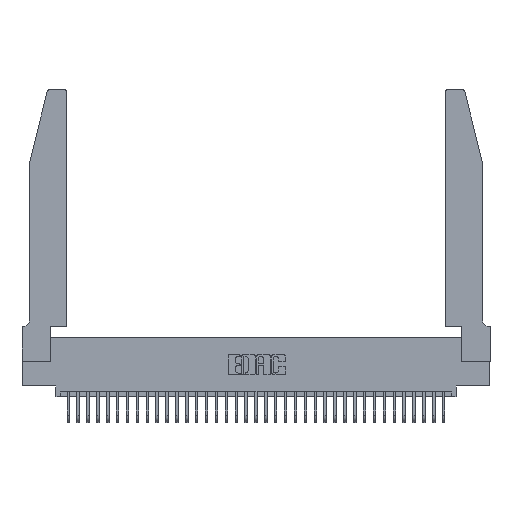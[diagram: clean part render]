
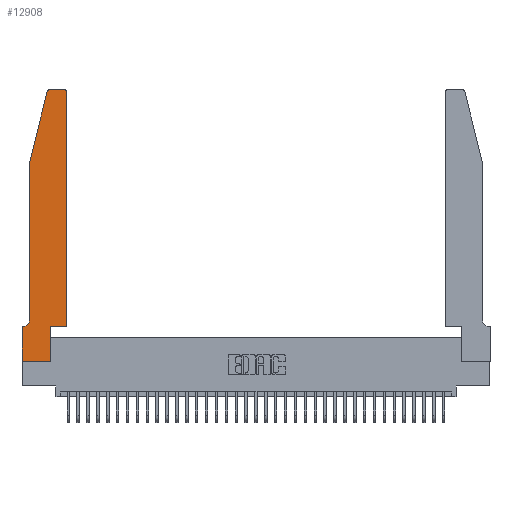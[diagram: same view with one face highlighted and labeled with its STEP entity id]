
A CAD part, top view. The second image highlights one B-rep face of the part: STEP entity #12908.
In plain terms, the highlighted planar face has unit normal (0, 0, 1).
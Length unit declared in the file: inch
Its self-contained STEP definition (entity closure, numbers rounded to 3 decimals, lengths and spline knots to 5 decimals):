
#141 = VERTEX_POINT ( 'NONE', #36667 ) ;
#667 = VERTEX_POINT ( 'NONE', #1172 ) ;
#768 = DIRECTION ( 'NONE',  ( -0.239, -0.971, 0. ) ) ;
#1172 = CARTESIAN_POINT ( 'NONE',  ( 0.4505, 2.72, 0.37 ) ) ;
#1260 = VECTOR ( 'NONE', #20683, 39.37008 ) ;
#2065 = CARTESIAN_POINT ( 'NONE',  ( 0.4205, 2.75, 0.37 ) ) ;
#2400 = EDGE_CURVE ( 'NONE', #3480, #141, #33584, .T. ) ;
#2544 = DIRECTION ( 'NONE',  ( 1., 0., 0. ) ) ;
#2602 = ORIENTED_EDGE ( 'NONE', *, *, #32186, .T. ) ;
#2661 = CARTESIAN_POINT ( 'NONE',  ( 0.4205, 2.72, 0.37 ) ) ;
#2886 = VERTEX_POINT ( 'NONE', #15798 ) ;
#3002 = LINE ( 'NONE', #16115, #18482 ) ;
#3480 = VERTEX_POINT ( 'NONE', #23937 ) ;
#3570 = ORIENTED_EDGE ( 'NONE', *, *, #16073, .T. ) ;
#3605 = CARTESIAN_POINT ( 'NONE',  ( 0.0755, 0.35, 0.37 ) ) ;
#4008 = ORIENTED_EDGE ( 'NONE', *, *, #9879, .T. ) ;
#4203 = LINE ( 'NONE', #15121, #12933 ) ;
#4409 = PLANE ( 'NONE',  #6894 ) ;
#4458 = CIRCLE ( 'NONE', #30157, 0.07 ) ;
#5718 = DIRECTION ( 'NONE',  ( 1., 0., 0. ) ) ;
#5922 = ORIENTED_EDGE ( 'NONE', *, *, #36748, .T. ) ;
#6076 = EDGE_CURVE ( 'NONE', #141, #10986, #3002, .T. ) ;
#6321 = CARTESIAN_POINT ( 'NONE',  ( 0.0755, 2., 0.37 ) ) ;
#6894 = AXIS2_PLACEMENT_3D ( 'NONE', #33172, #7443, #27545 ) ;
#7246 = EDGE_LOOP ( 'NONE', ( #5922, #22744, #2602, #20320, #26443, #3570, #18858, #15728, #10095, #23971, #4008, #20826 ) ) ;
#7443 = DIRECTION ( 'NONE',  ( 0., 0., 1. ) ) ;
#8031 = VECTOR ( 'NONE', #26484, 39.37008 ) ;
#8794 = CARTESIAN_POINT ( 'NONE',  ( 0.2605, 2.75, 0.37 ) ) ;
#9444 = EDGE_CURVE ( 'NONE', #35094, #15275, #4458, .T. ) ;
#9879 = EDGE_CURVE ( 'NONE', #30134, #667, #21654, .T. ) ;
#10061 = VERTEX_POINT ( 'NONE', #32057 ) ;
#10095 = ORIENTED_EDGE ( 'NONE', *, *, #6076, .T. ) ;
#10632 = EDGE_CURVE ( 'NONE', #667, #16925, #10797, .T. ) ;
#10673 = VECTOR ( 'NONE', #14799, 39.37008 ) ;
#10797 = CIRCLE ( 'NONE', #25418, 0.03 ) ;
#10986 = VERTEX_POINT ( 'NONE', #36030 ) ;
#11271 = CARTESIAN_POINT ( 'NONE',  ( 0.25487, 2.72718, 0.37 ) ) ;
#11391 = CARTESIAN_POINT ( 'NONE',  ( 0.0055, 0.42, 0.37 ) ) ;
#11578 = LINE ( 'NONE', #8794, #33580 ) ;
#11681 = DIRECTION ( 'NONE',  ( -1., 0., 0. ) ) ;
#12421 = VECTOR ( 'NONE', #32528, 39.37008 ) ;
#12908 = ADVANCED_FACE ( 'NONE', ( #35864 ), #4409, .T. ) ;
#12933 = VECTOR ( 'NONE', #35219, 39.37008 ) ;
#13266 = DIRECTION ( 'NONE',  ( 0., 1., 0. ) ) ;
#13899 = LINE ( 'NONE', #6321, #8031 ) ;
#14294 = DIRECTION ( 'NONE',  ( -1., 0., 0. ) ) ;
#14799 = DIRECTION ( 'NONE',  ( 1., 0., 0. ) ) ;
#15121 = CARTESIAN_POINT ( 'NONE',  ( 0.4505, 0.35, 0.37 ) ) ;
#15275 = VERTEX_POINT ( 'NONE', #17233 ) ;
#15431 = EDGE_CURVE ( 'NONE', #10986, #30134, #4203, .T. ) ;
#15728 = ORIENTED_EDGE ( 'NONE', *, *, #2400, .T. ) ;
#15798 = CARTESIAN_POINT ( 'NONE',  ( 0., 0.35, 0.37 ) ) ;
#16073 = EDGE_CURVE ( 'NONE', #15275, #2886, #27684, .T. ) ;
#16115 = CARTESIAN_POINT ( 'NONE',  ( 0.2865, 0.35, 0.37 ) ) ;
#16925 = VERTEX_POINT ( 'NONE', #2065 ) ;
#16990 = CARTESIAN_POINT ( 'NONE',  ( 0.4505, 0.35, 0.37 ) ) ;
#17233 = CARTESIAN_POINT ( 'NONE',  ( 0.0055, 0.35, 0.37 ) ) ;
#18482 = VECTOR ( 'NONE', #13266, 39.37008 ) ;
#18858 = ORIENTED_EDGE ( 'NONE', *, *, #22259, .T. ) ;
#19519 = VECTOR ( 'NONE', #768, 39.37008 ) ;
#19980 = DIRECTION ( 'NONE',  ( 0., 0., 1. ) ) ;
#20320 = ORIENTED_EDGE ( 'NONE', *, *, #29810, .T. ) ;
#20683 = DIRECTION ( 'NONE',  ( 0., -1., 0. ) ) ;
#20826 = ORIENTED_EDGE ( 'NONE', *, *, #10632, .T. ) ;
#21654 = LINE ( 'NONE', #27814, #27502 ) ;
#22042 = VERTEX_POINT ( 'NONE', #11271 ) ;
#22164 = DIRECTION ( 'NONE',  ( 0., 1., 0. ) ) ;
#22259 = EDGE_CURVE ( 'NONE', #2886, #3480, #32118, .T. ) ;
#22744 = ORIENTED_EDGE ( 'NONE', *, *, #33244, .T. ) ;
#22995 = DIRECTION ( 'NONE',  ( 0., 0., 1. ) ) ;
#23862 = CARTESIAN_POINT ( 'NONE',  ( 0.0755, 0.42, 0.37 ) ) ;
#23937 = CARTESIAN_POINT ( 'NONE',  ( 0., 0., 0.37 ) ) ;
#23971 = ORIENTED_EDGE ( 'NONE', *, *, #15431, .T. ) ;
#25418 = AXIS2_PLACEMENT_3D ( 'NONE', #2661, #22995, #5718 ) ;
#26443 = ORIENTED_EDGE ( 'NONE', *, *, #9444, .T. ) ;
#26484 = DIRECTION ( 'NONE',  ( 0., -1., 0. ) ) ;
#26877 = CARTESIAN_POINT ( 'NONE',  ( 0.0755, 2., 0.37 ) ) ;
#27502 = VECTOR ( 'NONE', #22164, 39.37008 ) ;
#27545 = DIRECTION ( 'NONE',  ( 1., 0., 0. ) ) ;
#27568 = VERTEX_POINT ( 'NONE', #29448 ) ;
#27684 = LINE ( 'NONE', #3605, #12421 ) ;
#27814 = CARTESIAN_POINT ( 'NONE',  ( 0.4505, 0.35, 0.37 ) ) ;
#29315 = CARTESIAN_POINT ( 'NONE',  ( 0., 0., 0.37 ) ) ;
#29448 = CARTESIAN_POINT ( 'NONE',  ( 0.0755, 2., 0.37 ) ) ;
#29810 = EDGE_CURVE ( 'NONE', #27568, #35094, #13899, .T. ) ;
#30134 = VERTEX_POINT ( 'NONE', #16990 ) ;
#30157 = AXIS2_PLACEMENT_3D ( 'NONE', #11391, #31480, #14294 ) ;
#31480 = DIRECTION ( 'NONE',  ( 0., 0., -1. ) ) ;
#32057 = CARTESIAN_POINT ( 'NONE',  ( 0.284, 2.75, 0.37 ) ) ;
#32118 = LINE ( 'NONE', #29315, #1260 ) ;
#32186 = EDGE_CURVE ( 'NONE', #22042, #27568, #34818, .T. ) ;
#32528 = DIRECTION ( 'NONE',  ( -1., 0., 0. ) ) ;
#33172 = CARTESIAN_POINT ( 'NONE',  ( 0., 0.35, 0.37 ) ) ;
#33244 = EDGE_CURVE ( 'NONE', #10061, #22042, #36571, .T. ) ;
#33580 = VECTOR ( 'NONE', #11681, 39.37008 ) ;
#33584 = LINE ( 'NONE', #34893, #10673 ) ;
#34818 = LINE ( 'NONE', #26877, #19519 ) ;
#34893 = CARTESIAN_POINT ( 'NONE',  ( 0., 0., 0.37 ) ) ;
#34932 = AXIS2_PLACEMENT_3D ( 'NONE', #37179, #19980, #2544 ) ;
#35094 = VERTEX_POINT ( 'NONE', #23862 ) ;
#35219 = DIRECTION ( 'NONE',  ( 1., 0., 0. ) ) ;
#35864 = FACE_OUTER_BOUND ( 'NONE', #7246, .T. ) ;
#36030 = CARTESIAN_POINT ( 'NONE',  ( 0.2865, 0.35, 0.37 ) ) ;
#36571 = CIRCLE ( 'NONE', #34932, 0.03 ) ;
#36667 = CARTESIAN_POINT ( 'NONE',  ( 0.2865, 0., 0.37 ) ) ;
#36748 = EDGE_CURVE ( 'NONE', #16925, #10061, #11578, .T. ) ;
#37179 = CARTESIAN_POINT ( 'NONE',  ( 0.284, 2.72, 0.37 ) ) ;
